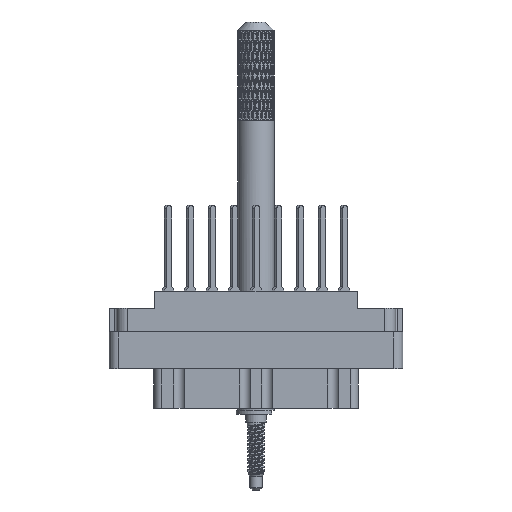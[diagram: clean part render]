
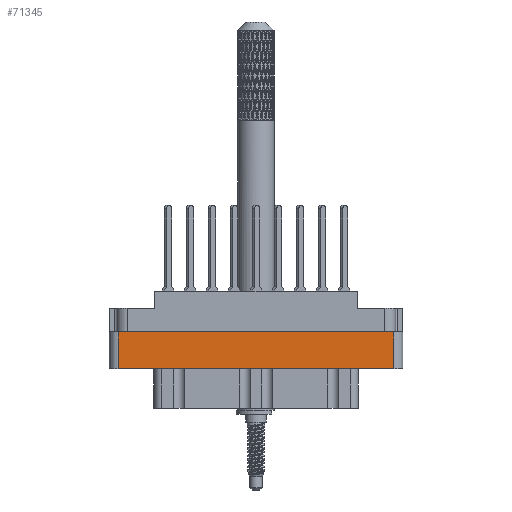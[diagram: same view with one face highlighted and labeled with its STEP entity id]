
A CAD part, front view. The second image highlights one B-rep face of the part: STEP entity #71345.
In plain terms, the highlighted planar face has unit normal (0, -1, 0).
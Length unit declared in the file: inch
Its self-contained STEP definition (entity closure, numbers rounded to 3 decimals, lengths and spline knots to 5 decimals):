
#2659 = CARTESIAN_POINT ( 'NONE',  ( -1., -0.438, -0.277 ) ) ;
#10296 = DIRECTION ( 'NONE',  ( 0., 0., 1. ) ) ;
#13912 = VECTOR ( 'NONE', #84027, 39.37008 ) ;
#14545 = EDGE_CURVE ( 'NONE', #70975, #78361, #69010, .T. ) ;
#16494 = ORIENTED_EDGE ( 'NONE', *, *, #91531, .T. ) ;
#16614 = EDGE_LOOP ( 'NONE', ( #75158, #29978, #16494, #94382 ) ) ;
#18005 = LINE ( 'NONE', #49507, #64955 ) ;
#25863 = LINE ( 'NONE', #2659, #74723 ) ;
#29978 = ORIENTED_EDGE ( 'NONE', *, *, #68055, .F. ) ;
#32932 = AXIS2_PLACEMENT_3D ( 'NONE', #72238, #34022, #88263 ) ;
#34022 = DIRECTION ( 'NONE',  ( 0., -1., 0. ) ) ;
#34661 = DIRECTION ( 'NONE',  ( 1., 0., 0. ) ) ;
#40724 = PLANE ( 'NONE',  #32932 ) ;
#42277 = FACE_OUTER_BOUND ( 'NONE', #16614, .T. ) ;
#45214 = CARTESIAN_POINT ( 'NONE',  ( 0.938, -0.438, -0.277 ) ) ;
#47748 = CARTESIAN_POINT ( 'NONE',  ( -0.938, -0.438, -0.277 ) ) ;
#47784 = CARTESIAN_POINT ( 'NONE',  ( 0.938, -0.438, -0.529 ) ) ;
#49507 = CARTESIAN_POINT ( 'NONE',  ( 0.938, -0.438, -0.798 ) ) ;
#54550 = CARTESIAN_POINT ( 'NONE',  ( -0.938, -0.438, -0.529 ) ) ;
#55233 = VERTEX_POINT ( 'NONE', #47784 ) ;
#60234 = LINE ( 'NONE', #92254, #75068 ) ;
#60827 = EDGE_CURVE ( 'NONE', #78361, #97683, #25863, .T. ) ;
#64955 = VECTOR ( 'NONE', #10296, 39.37008 ) ;
#68055 = EDGE_CURVE ( 'NONE', #55233, #70975, #60234, .T. ) ;
#69010 = LINE ( 'NONE', #100527, #13912 ) ;
#70975 = VERTEX_POINT ( 'NONE', #54550 ) ;
#71345 = ADVANCED_FACE ( 'NONE', ( #42277 ), #40724, .T. ) ;
#72238 = CARTESIAN_POINT ( 'NONE',  ( -0.938, -0.438, -0.798 ) ) ;
#74723 = VECTOR ( 'NONE', #34661, 39.37008 ) ;
#75068 = VECTOR ( 'NONE', #91769, 39.37008 ) ;
#75158 = ORIENTED_EDGE ( 'NONE', *, *, #14545, .F. ) ;
#78361 = VERTEX_POINT ( 'NONE', #47748 ) ;
#84027 = DIRECTION ( 'NONE',  ( 0., 0., 1. ) ) ;
#88263 = DIRECTION ( 'NONE',  ( 0., 0., -1. ) ) ;
#91531 = EDGE_CURVE ( 'NONE', #55233, #97683, #18005, .T. ) ;
#91769 = DIRECTION ( 'NONE',  ( -1., 0., 0. ) ) ;
#92254 = CARTESIAN_POINT ( 'NONE',  ( 0.938, -0.438, -0.529 ) ) ;
#94382 = ORIENTED_EDGE ( 'NONE', *, *, #60827, .F. ) ;
#97683 = VERTEX_POINT ( 'NONE', #45214 ) ;
#100527 = CARTESIAN_POINT ( 'NONE',  ( -0.938, -0.438, -0.798 ) ) ;
